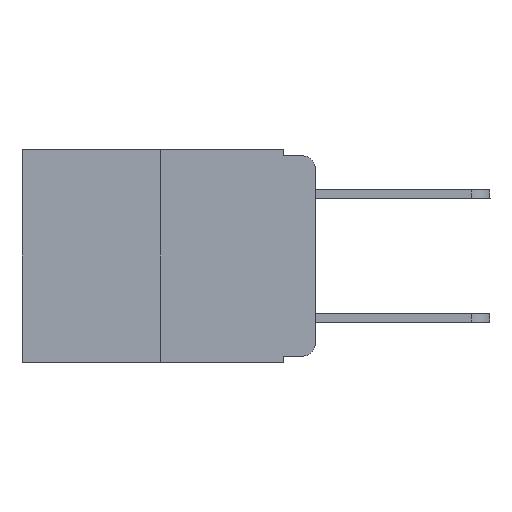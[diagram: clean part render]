
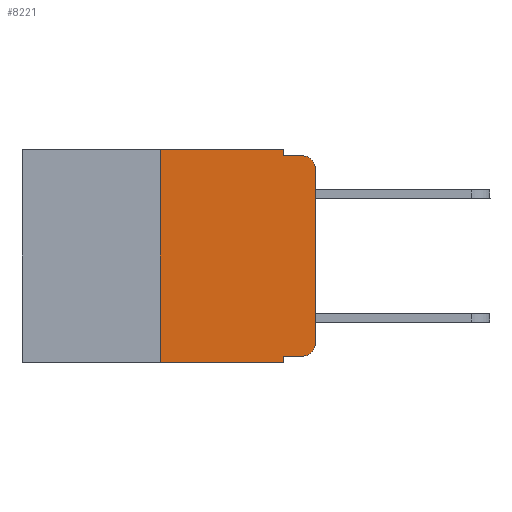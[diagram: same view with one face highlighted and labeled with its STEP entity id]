
A CAD part, left-side view. The second image highlights one B-rep face of the part: STEP entity #8221.
In plain terms, the highlighted planar face has unit normal (-1, 0, 0).
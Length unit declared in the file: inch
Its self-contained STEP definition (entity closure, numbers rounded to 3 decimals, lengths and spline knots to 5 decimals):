
#158 = DIRECTION ( 'NONE',  ( 0., 0., 1. ) ) ;
#452 = EDGE_CURVE ( 'NONE', #10934, #3448, #3474, .T. ) ;
#463 = LINE ( 'NONE', #16265, #11481 ) ;
#492 = CARTESIAN_POINT ( 'NONE',  ( 0., 0.25, 0. ) ) ;
#1302 = CARTESIAN_POINT ( 'NONE',  ( 0., 0.051, -0.333 ) ) ;
#1334 = VERTEX_POINT ( 'NONE', #5286 ) ;
#1400 = CARTESIAN_POINT ( 'NONE',  ( 0., 0.473, 0. ) ) ;
#1497 = ORIENTED_EDGE ( 'NONE', *, *, #452, .F. ) ;
#1917 = DIRECTION ( 'NONE',  ( 0., -1., 0. ) ) ;
#1921 = VECTOR ( 'NONE', #11939, 39.37008 ) ;
#2273 = CARTESIAN_POINT ( 'NONE',  ( 0., 0.02, -0.03 ) ) ;
#3271 = DIRECTION ( 'NONE',  ( 0., 0., -1. ) ) ;
#3448 = VERTEX_POINT ( 'NONE', #15815 ) ;
#3474 = LINE ( 'NONE', #6484, #12765 ) ;
#4296 = DIRECTION ( 'NONE',  ( 0., 0., -1. ) ) ;
#4562 = DIRECTION ( 'NONE',  ( 1., 0., 0. ) ) ;
#4761 = DIRECTION ( 'NONE',  ( 0., -1., 0. ) ) ;
#5286 = CARTESIAN_POINT ( 'NONE',  ( 0., 0.02, -0.01 ) ) ;
#5454 = DIRECTION ( 'NONE',  ( 0., 0., -1. ) ) ;
#5501 = CARTESIAN_POINT ( 'NONE',  ( 0., 0.02, -0.333 ) ) ;
#5711 = ORIENTED_EDGE ( 'NONE', *, *, #12027, .F. ) ;
#5865 = CARTESIAN_POINT ( 'NONE',  ( 0., 0.473, 0. ) ) ;
#6123 = EDGE_CURVE ( 'NONE', #10934, #13670, #463, .T. ) ;
#6381 = DIRECTION ( 'NONE',  ( 0., -1., 0. ) ) ;
#6462 = CARTESIAN_POINT ( 'NONE',  ( 0., 0.051, -0.01 ) ) ;
#6484 = CARTESIAN_POINT ( 'NONE',  ( 0., 0.051, 0. ) ) ;
#6723 = CARTESIAN_POINT ( 'NONE',  ( 0., 0.25, -0.343 ) ) ;
#6762 = VERTEX_POINT ( 'NONE', #15988 ) ;
#6988 = ORIENTED_EDGE ( 'NONE', *, *, #11264, .F. ) ;
#7122 = CARTESIAN_POINT ( 'NONE',  ( 0., 0.051, 0. ) ) ;
#7295 = LINE ( 'NONE', #7122, #14372 ) ;
#7403 = DIRECTION ( 'NONE',  ( 0., 0., -1. ) ) ;
#8027 = LINE ( 'NONE', #6462, #10436 ) ;
#8111 = EDGE_CURVE ( 'NONE', #9478, #6762, #15197, .T. ) ;
#8162 = ORIENTED_EDGE ( 'NONE', *, *, #14361, .T. ) ;
#8221 = ADVANCED_FACE ( 'NONE', ( #8649 ), #11209, .F. ) ;
#8275 = DIRECTION ( 'NONE',  ( -1., 0., 0. ) ) ;
#8346 = LINE ( 'NONE', #16854, #11245 ) ;
#8453 = VERTEX_POINT ( 'NONE', #13371 ) ;
#8507 = EDGE_CURVE ( 'NONE', #13670, #9478, #17022, .T. ) ;
#8649 = FACE_OUTER_BOUND ( 'NONE', #9671, .T. ) ;
#8724 = CARTESIAN_POINT ( 'NONE',  ( 0., 0., 0. ) ) ;
#9169 = EDGE_CURVE ( 'NONE', #9932, #3448, #8346, .T. ) ;
#9478 = VERTEX_POINT ( 'NONE', #14861 ) ;
#9671 = EDGE_LOOP ( 'NONE', ( #16669, #8162, #14022, #5711, #6988, #14026, #16165, #1497, #11502, #15680 ) ) ;
#9742 = EDGE_CURVE ( 'NONE', #8453, #1334, #8027, .T. ) ;
#9932 = VERTEX_POINT ( 'NONE', #6723 ) ;
#10436 = VECTOR ( 'NONE', #6381, 39.37008 ) ;
#10679 = AXIS2_PLACEMENT_3D ( 'NONE', #5865, #4562, #7403 ) ;
#10869 = VERTEX_POINT ( 'NONE', #14432 ) ;
#10934 = VERTEX_POINT ( 'NONE', #1302 ) ;
#10979 = CIRCLE ( 'NONE', #11522, 0.02 ) ;
#11209 = PLANE ( 'NONE',  #10679 ) ;
#11245 = VECTOR ( 'NONE', #4761, 39.37008 ) ;
#11264 = EDGE_CURVE ( 'NONE', #15028, #10869, #14603, .T. ) ;
#11296 = DIRECTION ( 'NONE',  ( 0., 0., 1. ) ) ;
#11415 = DIRECTION ( 'NONE',  ( 0., 0., -1. ) ) ;
#11481 = VECTOR ( 'NONE', #1917, 39.37008 ) ;
#11502 = ORIENTED_EDGE ( 'NONE', *, *, #6123, .T. ) ;
#11522 = AXIS2_PLACEMENT_3D ( 'NONE', #2273, #11597, #11415 ) ;
#11597 = DIRECTION ( 'NONE',  ( -1., 0., 0. ) ) ;
#11939 = DIRECTION ( 'NONE',  ( 0., -1., 0. ) ) ;
#12027 = EDGE_CURVE ( 'NONE', #10869, #8453, #7295, .T. ) ;
#12327 = LINE ( 'NONE', #492, #14648 ) ;
#12765 = VECTOR ( 'NONE', #5454, 39.37008 ) ;
#13371 = CARTESIAN_POINT ( 'NONE',  ( 0., 0.051, -0.01 ) ) ;
#13617 = CARTESIAN_POINT ( 'NONE',  ( 0., 0.02, -0.313 ) ) ;
#13670 = VERTEX_POINT ( 'NONE', #5501 ) ;
#13705 = VECTOR ( 'NONE', #11296, 39.37008 ) ;
#14022 = ORIENTED_EDGE ( 'NONE', *, *, #9742, .F. ) ;
#14026 = ORIENTED_EDGE ( 'NONE', *, *, #16673, .F. ) ;
#14361 = EDGE_CURVE ( 'NONE', #6762, #1334, #10979, .T. ) ;
#14372 = VECTOR ( 'NONE', #3271, 39.37008 ) ;
#14432 = CARTESIAN_POINT ( 'NONE',  ( 0., 0.051, 0. ) ) ;
#14603 = LINE ( 'NONE', #1400, #1921 ) ;
#14648 = VECTOR ( 'NONE', #158, 39.37008 ) ;
#14861 = CARTESIAN_POINT ( 'NONE',  ( 0., 0., -0.313 ) ) ;
#15028 = VERTEX_POINT ( 'NONE', #16533 ) ;
#15197 = LINE ( 'NONE', #8724, #13705 ) ;
#15361 = AXIS2_PLACEMENT_3D ( 'NONE', #13617, #8275, #4296 ) ;
#15680 = ORIENTED_EDGE ( 'NONE', *, *, #8507, .T. ) ;
#15815 = CARTESIAN_POINT ( 'NONE',  ( 0., 0.051, -0.343 ) ) ;
#15988 = CARTESIAN_POINT ( 'NONE',  ( 0., 0., -0.03 ) ) ;
#16165 = ORIENTED_EDGE ( 'NONE', *, *, #9169, .T. ) ;
#16265 = CARTESIAN_POINT ( 'NONE',  ( 0., 0.051, -0.333 ) ) ;
#16533 = CARTESIAN_POINT ( 'NONE',  ( 0., 0.25, 0. ) ) ;
#16669 = ORIENTED_EDGE ( 'NONE', *, *, #8111, .T. ) ;
#16673 = EDGE_CURVE ( 'NONE', #9932, #15028, #12327, .T. ) ;
#16854 = CARTESIAN_POINT ( 'NONE',  ( 0., 0.473, -0.343 ) ) ;
#17022 = CIRCLE ( 'NONE', #15361, 0.02 ) ;
